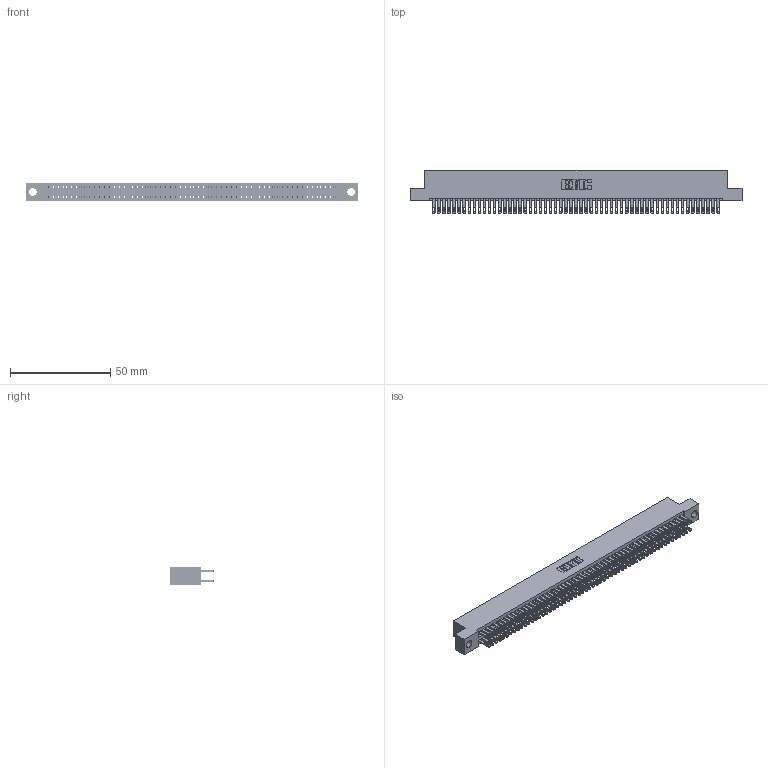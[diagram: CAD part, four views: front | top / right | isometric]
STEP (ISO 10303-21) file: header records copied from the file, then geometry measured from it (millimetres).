
FILE_DESCRIPTION (( 'STEP AP203' ), '1' );
FILE_NAME ('345-114-500-204.STEP', '2021-05-25T14:48:57', ( '' ), ( '' ), 'SwSTEP 2.0', 'SolidWorks 2020', '' );
FILE_SCHEMA (( 'CONFIG_CONTROL_DESIGN' ));
Length unit declared in the file: inch
Products named in the file (3): 345-292-001_345-293-100; 345-114-500-204; 345 Part_Flush Mounting Lugs - 0.156 Dia-TI
Assembly tree (115 placements, depth 2):
  345-114-500-204
    345 Part_Flush Mounting Lugs - 0.156 Dia-TI
    345-292-001_345-293-100  x114
Bounding box: 165.99 x 21.51 x 9.4 mm (x, y, z)
Volume: 16506 mm3; surface area: 25703.5 mm2
Topology: 115 solids, 115 shells, 5384 faces, 16451 edges, 10966 vertices
Faces by surface type: plane 3172, cylinder 2212
Entity records: 43053 total; most frequent: CARTESIAN_POINT 7206, ORIENTED_EDGE 7138, DIRECTION 6337, EDGE_CURVE 3569, LINE 3205, VECTOR 3205, VERTEX_POINT 2378, AXIS2_PLACEMENT_3D 1566
